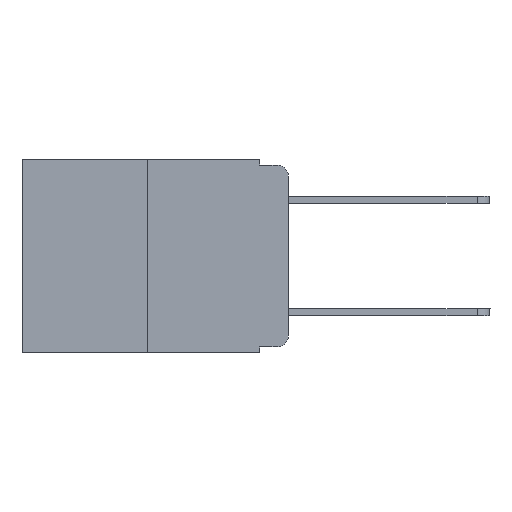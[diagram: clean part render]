
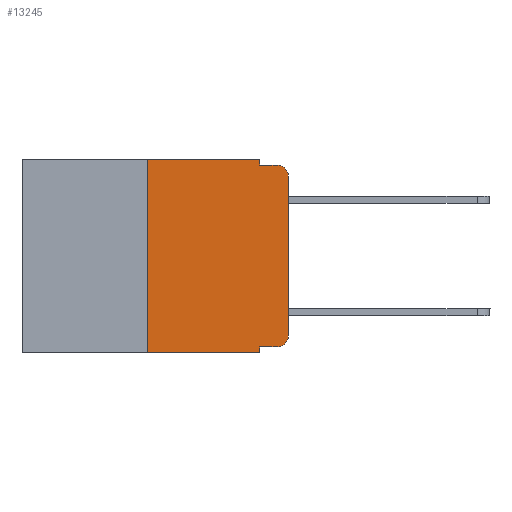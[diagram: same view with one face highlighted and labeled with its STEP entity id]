
A CAD part, left-side view. The second image highlights one B-rep face of the part: STEP entity #13245.
In plain terms, the highlighted planar face has unit normal (-1, 0, 0).
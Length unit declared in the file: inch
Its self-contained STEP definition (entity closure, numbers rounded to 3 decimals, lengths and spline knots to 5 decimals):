
#111 = VERTEX_POINT ( 'NONE', #13755 ) ;
#263 = CIRCLE ( 'NONE', #541, 0.02 ) ;
#395 = ORIENTED_EDGE ( 'NONE', *, *, #9688, .T. ) ;
#541 = AXIS2_PLACEMENT_3D ( 'NONE', #9747, #16483, #3515 ) ;
#718 = CARTESIAN_POINT ( 'NONE',  ( 0., 0.473, 0. ) ) ;
#982 = VERTEX_POINT ( 'NONE', #6856 ) ;
#1047 = CARTESIAN_POINT ( 'NONE',  ( 0., 0.051, -0.343 ) ) ;
#1397 = AXIS2_PLACEMENT_3D ( 'NONE', #10155, #15198, #3329 ) ;
#1461 = CARTESIAN_POINT ( 'NONE',  ( 0., 0.051, 0. ) ) ;
#1477 = VERTEX_POINT ( 'NONE', #5355 ) ;
#1729 = LINE ( 'NONE', #4325, #3730 ) ;
#2088 = VECTOR ( 'NONE', #15046, 39.37008 ) ;
#2531 = CARTESIAN_POINT ( 'NONE',  ( 0., 0.051, -0.01 ) ) ;
#2688 = CARTESIAN_POINT ( 'NONE',  ( 0., 0.25, 0. ) ) ;
#2759 = CARTESIAN_POINT ( 'NONE',  ( 0., 0., -0.03 ) ) ;
#2985 = LINE ( 'NONE', #11519, #14243 ) ;
#2996 = DIRECTION ( 'NONE',  ( 0., -1., 0. ) ) ;
#3095 = DIRECTION ( 'NONE',  ( 0., 0., -1. ) ) ;
#3329 = DIRECTION ( 'NONE',  ( 0., 0., -1. ) ) ;
#3435 = CARTESIAN_POINT ( 'NONE',  ( 0., 0.473, -0.343 ) ) ;
#3515 = DIRECTION ( 'NONE',  ( 0., 0., -1. ) ) ;
#3614 = EDGE_CURVE ( 'NONE', #12241, #11767, #2985, .T. ) ;
#3730 = VECTOR ( 'NONE', #8396, 39.37008 ) ;
#3904 = VERTEX_POINT ( 'NONE', #1047 ) ;
#4128 = VERTEX_POINT ( 'NONE', #2759 ) ;
#4325 = CARTESIAN_POINT ( 'NONE',  ( 0., 0., 0. ) ) ;
#4351 = EDGE_CURVE ( 'NONE', #1477, #3904, #5335, .T. ) ;
#4361 = VECTOR ( 'NONE', #10060, 39.37008 ) ;
#4387 = CARTESIAN_POINT ( 'NONE',  ( 0., 0.051, 0. ) ) ;
#4417 = EDGE_LOOP ( 'NONE', ( #6076, #395, #6282, #4698, #8490, #14201, #4782, #5732, #11659, #6193 ) ) ;
#4694 = DIRECTION ( 'NONE',  ( 1., 0., 0. ) ) ;
#4698 = ORIENTED_EDGE ( 'NONE', *, *, #13996, .F. ) ;
#4726 = VECTOR ( 'NONE', #16011, 39.37008 ) ;
#4782 = ORIENTED_EDGE ( 'NONE', *, *, #4351, .T. ) ;
#5335 = LINE ( 'NONE', #3435, #2088 ) ;
#5355 = CARTESIAN_POINT ( 'NONE',  ( 0., 0.25, -0.343 ) ) ;
#5396 = CARTESIAN_POINT ( 'NONE',  ( 0., 0.051, -0.333 ) ) ;
#5732 = ORIENTED_EDGE ( 'NONE', *, *, #12160, .F. ) ;
#6055 = DIRECTION ( 'NONE',  ( 0., -1., 0. ) ) ;
#6076 = ORIENTED_EDGE ( 'NONE', *, *, #15212, .T. ) ;
#6193 = ORIENTED_EDGE ( 'NONE', *, *, #11531, .T. ) ;
#6282 = ORIENTED_EDGE ( 'NONE', *, *, #7883, .F. ) ;
#6856 = CARTESIAN_POINT ( 'NONE',  ( 0., 0.02, -0.333 ) ) ;
#7883 = EDGE_CURVE ( 'NONE', #13734, #14499, #8763, .T. ) ;
#8396 = DIRECTION ( 'NONE',  ( 0., 0., 1. ) ) ;
#8490 = ORIENTED_EDGE ( 'NONE', *, *, #3614, .F. ) ;
#8605 = CARTESIAN_POINT ( 'NONE',  ( 0., 0.02, -0.01 ) ) ;
#8763 = LINE ( 'NONE', #2531, #4361 ) ;
#9086 = CARTESIAN_POINT ( 'NONE',  ( 0., 0.051, -0.01 ) ) ;
#9147 = CARTESIAN_POINT ( 'NONE',  ( 0., 0.25, 0. ) ) ;
#9300 = LINE ( 'NONE', #5396, #14995 ) ;
#9426 = EDGE_CURVE ( 'NONE', #1477, #12241, #11843, .T. ) ;
#9517 = VECTOR ( 'NONE', #3095, 39.37008 ) ;
#9625 = VERTEX_POINT ( 'NONE', #10713 ) ;
#9688 = EDGE_CURVE ( 'NONE', #4128, #14499, #263, .T. ) ;
#9747 = CARTESIAN_POINT ( 'NONE',  ( 0., 0.02, -0.03 ) ) ;
#9985 = DIRECTION ( 'NONE',  ( 0., 0., -1. ) ) ;
#10060 = DIRECTION ( 'NONE',  ( 0., -1., 0. ) ) ;
#10155 = CARTESIAN_POINT ( 'NONE',  ( 0., 0.02, -0.313 ) ) ;
#10713 = CARTESIAN_POINT ( 'NONE',  ( 0., 0., -0.313 ) ) ;
#11519 = CARTESIAN_POINT ( 'NONE',  ( 0., 0.473, 0. ) ) ;
#11531 = EDGE_CURVE ( 'NONE', #982, #9625, #16320, .T. ) ;
#11659 = ORIENTED_EDGE ( 'NONE', *, *, #12912, .T. ) ;
#11767 = VERTEX_POINT ( 'NONE', #13275 ) ;
#11843 = LINE ( 'NONE', #9147, #15462 ) ;
#12160 = EDGE_CURVE ( 'NONE', #111, #3904, #14816, .T. ) ;
#12241 = VERTEX_POINT ( 'NONE', #2688 ) ;
#12587 = PLANE ( 'NONE',  #15549 ) ;
#12912 = EDGE_CURVE ( 'NONE', #111, #982, #9300, .T. ) ;
#13245 = ADVANCED_FACE ( 'NONE', ( #15196 ), #12587, .F. ) ;
#13275 = CARTESIAN_POINT ( 'NONE',  ( 0., 0.051, 0. ) ) ;
#13734 = VERTEX_POINT ( 'NONE', #9086 ) ;
#13755 = CARTESIAN_POINT ( 'NONE',  ( 0., 0.051, -0.333 ) ) ;
#13996 = EDGE_CURVE ( 'NONE', #11767, #13734, #16243, .T. ) ;
#14201 = ORIENTED_EDGE ( 'NONE', *, *, #9426, .F. ) ;
#14243 = VECTOR ( 'NONE', #6055, 39.37008 ) ;
#14499 = VERTEX_POINT ( 'NONE', #8605 ) ;
#14816 = LINE ( 'NONE', #1461, #4726 ) ;
#14995 = VECTOR ( 'NONE', #2996, 39.37008 ) ;
#15046 = DIRECTION ( 'NONE',  ( 0., -1., 0. ) ) ;
#15196 = FACE_OUTER_BOUND ( 'NONE', #4417, .T. ) ;
#15198 = DIRECTION ( 'NONE',  ( -1., 0., 0. ) ) ;
#15212 = EDGE_CURVE ( 'NONE', #9625, #4128, #1729, .T. ) ;
#15462 = VECTOR ( 'NONE', #15556, 39.37008 ) ;
#15549 = AXIS2_PLACEMENT_3D ( 'NONE', #718, #4694, #9985 ) ;
#15556 = DIRECTION ( 'NONE',  ( 0., 0., 1. ) ) ;
#16011 = DIRECTION ( 'NONE',  ( 0., 0., -1. ) ) ;
#16243 = LINE ( 'NONE', #4387, #9517 ) ;
#16320 = CIRCLE ( 'NONE', #1397, 0.02 ) ;
#16483 = DIRECTION ( 'NONE',  ( -1., 0., 0. ) ) ;
